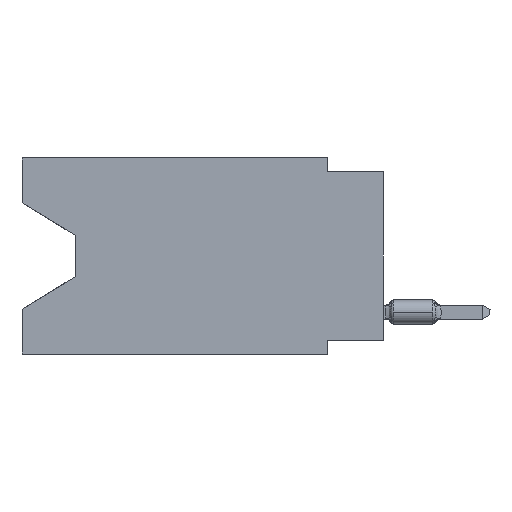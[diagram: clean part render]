
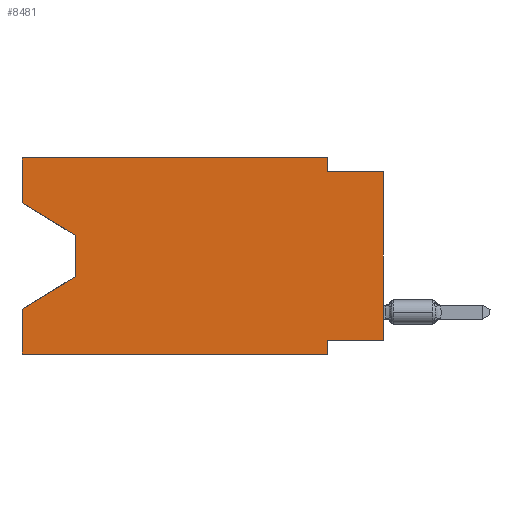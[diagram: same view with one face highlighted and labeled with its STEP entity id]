
A CAD part, left-side view. The second image highlights one B-rep face of the part: STEP entity #8481.
In plain terms, the highlighted planar face has unit normal (-1, 0, 0).
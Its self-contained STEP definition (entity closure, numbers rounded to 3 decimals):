
#140 = ORIENTED_EDGE ( 'NONE', *, *, #30302, .T. ) ;
#228 = LINE ( 'NONE', #5632, #20113 ) ;
#898 = CARTESIAN_POINT ( 'NONE',  ( 0., 16.383, 0. ) ) ;
#1320 = LINE ( 'NONE', #12646, #26937 ) ;
#2034 = EDGE_CURVE ( 'NONE', #16840, #30418, #19128, .T. ) ;
#2623 = EDGE_LOOP ( 'NONE', ( #140, #16732, #9698, #8416, #5408, #17641, #19297, #29158, #21500, #35632, #32448, #34388 ) ) ;
#2803 = CARTESIAN_POINT ( 'NONE',  ( 0., 0., 0. ) ) ;
#3142 = DIRECTION ( 'NONE',  ( 0., 0.855, -0.519 ) ) ;
#3176 = CARTESIAN_POINT ( 'NONE',  ( 0., 16.383, 0. ) ) ;
#4032 = CARTESIAN_POINT ( 'NONE',  ( 0., 13.97, -3.505 ) ) ;
#4224 = CARTESIAN_POINT ( 'NONE',  ( 0., 2.54, 0. ) ) ;
#5408 = ORIENTED_EDGE ( 'NONE', *, *, #22768, .T. ) ;
#5632 = CARTESIAN_POINT ( 'NONE',  ( 0., 13.97, -3.505 ) ) ;
#6196 = LINE ( 'NONE', #20311, #15170 ) ;
#6478 = CARTESIAN_POINT ( 'NONE',  ( 0., 2.54, -8.255 ) ) ;
#6618 = CARTESIAN_POINT ( 'NONE',  ( 0., 0., -0.635 ) ) ;
#7033 = CARTESIAN_POINT ( 'NONE',  ( 0., 0., -8.255 ) ) ;
#7312 = CARTESIAN_POINT ( 'NONE',  ( 0., 16.383, -2.038 ) ) ;
#8198 = DIRECTION ( 'NONE',  ( 0., -1., 0. ) ) ;
#8242 = EDGE_CURVE ( 'NONE', #12147, #31184, #20241, .T. ) ;
#8416 = ORIENTED_EDGE ( 'NONE', *, *, #2034, .F. ) ;
#8481 = ADVANCED_FACE ( 'NONE', ( #9267 ), #26327, .F. ) ;
#8901 = DIRECTION ( 'NONE',  ( 0., -1., 0. ) ) ;
#9030 = DIRECTION ( 'NONE',  ( 0., 1., 0. ) ) ;
#9202 = EDGE_CURVE ( 'NONE', #21576, #31184, #25799, .T. ) ;
#9267 = FACE_OUTER_BOUND ( 'NONE', #2623, .T. ) ;
#9514 = CARTESIAN_POINT ( 'NONE',  ( 0., 2.54, 0. ) ) ;
#9576 = EDGE_CURVE ( 'NONE', #12147, #28069, #12200, .T. ) ;
#9698 = ORIENTED_EDGE ( 'NONE', *, *, #27965, .T. ) ;
#9793 = VERTEX_POINT ( 'NONE', #4032 ) ;
#10203 = VECTOR ( 'NONE', #25242, 1000. ) ;
#10258 = VERTEX_POINT ( 'NONE', #16216 ) ;
#11155 = VECTOR ( 'NONE', #9030, 1000. ) ;
#11350 = VERTEX_POINT ( 'NONE', #32707 ) ;
#11628 = AXIS2_PLACEMENT_3D ( 'NONE', #898, #20766, #20229 ) ;
#11673 = CARTESIAN_POINT ( 'NONE',  ( 0., 2.54, -0.635 ) ) ;
#11732 = LINE ( 'NONE', #3176, #17984 ) ;
#11954 = DIRECTION ( 'NONE',  ( 0., 0., -1. ) ) ;
#12147 = VERTEX_POINT ( 'NONE', #7033 ) ;
#12200 = LINE ( 'NONE', #19822, #11155 ) ;
#12646 = CARTESIAN_POINT ( 'NONE',  ( 0., 16.383, -2.038 ) ) ;
#12980 = CARTESIAN_POINT ( 'NONE',  ( 0., 13.97, -5.385 ) ) ;
#13958 = EDGE_CURVE ( 'NONE', #28069, #10258, #6196, .T. ) ;
#14238 = VECTOR ( 'NONE', #16649, 1000. ) ;
#14723 = VECTOR ( 'NONE', #3142, 1000. ) ;
#14954 = EDGE_CURVE ( 'NONE', #23432, #21576, #23802, .T. ) ;
#15170 = VECTOR ( 'NONE', #11954, 1000. ) ;
#15201 = EDGE_CURVE ( 'NONE', #11350, #23432, #11732, .T. ) ;
#16216 = CARTESIAN_POINT ( 'NONE',  ( 0., 2.54, -8.89 ) ) ;
#16649 = DIRECTION ( 'NONE',  ( 0., 0., 1. ) ) ;
#16732 = ORIENTED_EDGE ( 'NONE', *, *, #35422, .T. ) ;
#16840 = VERTEX_POINT ( 'NONE', #30247 ) ;
#17641 = ORIENTED_EDGE ( 'NONE', *, *, #13958, .F. ) ;
#17984 = VECTOR ( 'NONE', #8198, 1000. ) ;
#18764 = VECTOR ( 'NONE', #30810, 1000. ) ;
#19128 = LINE ( 'NONE', #30979, #10203 ) ;
#19136 = CARTESIAN_POINT ( 'NONE',  ( 0., 16.383, -6.852 ) ) ;
#19297 = ORIENTED_EDGE ( 'NONE', *, *, #9576, .F. ) ;
#19822 = CARTESIAN_POINT ( 'NONE',  ( 0., 0., -8.255 ) ) ;
#20113 = VECTOR ( 'NONE', #22703, 1000. ) ;
#20229 = DIRECTION ( 'NONE',  ( 0., 0., -1. ) ) ;
#20241 = LINE ( 'NONE', #2803, #18764 ) ;
#20311 = CARTESIAN_POINT ( 'NONE',  ( 0., 2.54, -8.89 ) ) ;
#20619 = VECTOR ( 'NONE', #8901, 1000. ) ;
#20766 = DIRECTION ( 'NONE',  ( 1., 0., 0. ) ) ;
#21500 = ORIENTED_EDGE ( 'NONE', *, *, #9202, .F. ) ;
#21520 = VECTOR ( 'NONE', #23631, 1000. ) ;
#21576 = VERTEX_POINT ( 'NONE', #11673 ) ;
#21757 = DIRECTION ( 'NONE',  ( 0., -0.855, -0.519 ) ) ;
#22703 = DIRECTION ( 'NONE',  ( 0., 0., -1. ) ) ;
#22768 = EDGE_CURVE ( 'NONE', #16840, #10258, #27552, .T. ) ;
#23432 = VERTEX_POINT ( 'NONE', #4224 ) ;
#23631 = DIRECTION ( 'NONE',  ( 0., 0., -1. ) ) ;
#23802 = LINE ( 'NONE', #9514, #21520 ) ;
#25242 = DIRECTION ( 'NONE',  ( 0., 0., 1. ) ) ;
#25799 = LINE ( 'NONE', #34327, #20619 ) ;
#26327 = PLANE ( 'NONE',  #11628 ) ;
#26937 = VECTOR ( 'NONE', #21757, 1000. ) ;
#27513 = VERTEX_POINT ( 'NONE', #7312 ) ;
#27552 = LINE ( 'NONE', #35516, #31700 ) ;
#27965 = EDGE_CURVE ( 'NONE', #29371, #30418, #28588, .T. ) ;
#28069 = VERTEX_POINT ( 'NONE', #6478 ) ;
#28588 = LINE ( 'NONE', #28953, #14723 ) ;
#28953 = CARTESIAN_POINT ( 'NONE',  ( 0., 13.97, -5.385 ) ) ;
#29158 = ORIENTED_EDGE ( 'NONE', *, *, #8242, .T. ) ;
#29371 = VERTEX_POINT ( 'NONE', #12980 ) ;
#30247 = CARTESIAN_POINT ( 'NONE',  ( 0., 16.383, -8.89 ) ) ;
#30302 = EDGE_CURVE ( 'NONE', #27513, #9793, #1320, .T. ) ;
#30418 = VERTEX_POINT ( 'NONE', #19136 ) ;
#30744 = LINE ( 'NONE', #34067, #14238 ) ;
#30810 = DIRECTION ( 'NONE',  ( 0., 0., 1. ) ) ;
#30979 = CARTESIAN_POINT ( 'NONE',  ( 0., 16.383, 0. ) ) ;
#31184 = VERTEX_POINT ( 'NONE', #6618 ) ;
#31700 = VECTOR ( 'NONE', #35694, 1000. ) ;
#32448 = ORIENTED_EDGE ( 'NONE', *, *, #15201, .F. ) ;
#32707 = CARTESIAN_POINT ( 'NONE',  ( 0., 16.383, 0. ) ) ;
#34067 = CARTESIAN_POINT ( 'NONE',  ( 0., 16.383, 0. ) ) ;
#34327 = CARTESIAN_POINT ( 'NONE',  ( 0., 0., -0.635 ) ) ;
#34388 = ORIENTED_EDGE ( 'NONE', *, *, #36331, .F. ) ;
#35422 = EDGE_CURVE ( 'NONE', #9793, #29371, #228, .T. ) ;
#35516 = CARTESIAN_POINT ( 'NONE',  ( 0., 16.383, -8.89 ) ) ;
#35632 = ORIENTED_EDGE ( 'NONE', *, *, #14954, .F. ) ;
#35694 = DIRECTION ( 'NONE',  ( 0., -1., 0. ) ) ;
#36331 = EDGE_CURVE ( 'NONE', #27513, #11350, #30744, .T. ) ;
